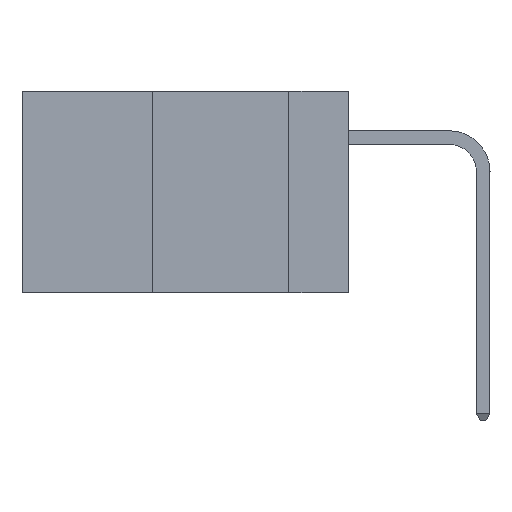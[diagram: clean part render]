
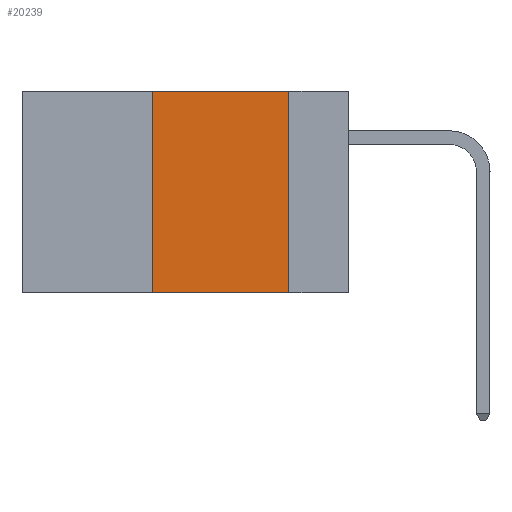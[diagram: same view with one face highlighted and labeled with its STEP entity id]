
A CAD part, left-side view. The second image highlights one B-rep face of the part: STEP entity #20239.
In plain terms, the highlighted planar face has unit normal (-1, 0, 0).
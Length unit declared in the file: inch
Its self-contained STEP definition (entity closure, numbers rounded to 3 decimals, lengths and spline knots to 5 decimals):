
#16 = CARTESIAN_POINT ( 'NONE',  ( 0., 0.11, 0. ) ) ;
#1268 = ORIENTED_EDGE ( 'NONE', *, *, #2205, .T. ) ;
#1293 = CARTESIAN_POINT ( 'NONE',  ( 0., 0.6, 0. ) ) ;
#1580 = EDGE_CURVE ( 'NONE', #20845, #8998, #15864, .T. ) ;
#2205 = EDGE_CURVE ( 'NONE', #19623, #19087, #8389, .T. ) ;
#2544 = EDGE_LOOP ( 'NONE', ( #24958, #12307, #13071, #1268 ) ) ;
#2777 = VECTOR ( 'NONE', #11764, 39.37008 ) ;
#3523 = DIRECTION ( 'NONE',  ( 0., 0., -1. ) ) ;
#3656 = PLANE ( 'NONE',  #23355 ) ;
#4199 = VECTOR ( 'NONE', #5696, 39.37008 ) ;
#5696 = DIRECTION ( 'NONE',  ( 0., -1., 0. ) ) ;
#7130 = EDGE_CURVE ( 'NONE', #8998, #19087, #12029, .T. ) ;
#8389 = LINE ( 'NONE', #16970, #13933 ) ;
#8667 = CARTESIAN_POINT ( 'NONE',  ( 0., 0.11, -0.37 ) ) ;
#8998 = VERTEX_POINT ( 'NONE', #13156 ) ;
#10999 = CARTESIAN_POINT ( 'NONE',  ( 0., 0.36, 0. ) ) ;
#11764 = DIRECTION ( 'NONE',  ( 0., 0., -1. ) ) ;
#12029 = LINE ( 'NONE', #16, #2777 ) ;
#12307 = ORIENTED_EDGE ( 'NONE', *, *, #1580, .F. ) ;
#13071 = ORIENTED_EDGE ( 'NONE', *, *, #18380, .F. ) ;
#13110 = DIRECTION ( 'NONE',  ( 0., 0., 1. ) ) ;
#13156 = CARTESIAN_POINT ( 'NONE',  ( 0., 0.11, 0. ) ) ;
#13695 = FACE_OUTER_BOUND ( 'NONE', #2544, .T. ) ;
#13933 = VECTOR ( 'NONE', #20390, 39.37008 ) ;
#14174 = CARTESIAN_POINT ( 'NONE',  ( 0., 0.36, -0.37 ) ) ;
#15101 = CARTESIAN_POINT ( 'NONE',  ( 0., 0.36, 0. ) ) ;
#15864 = LINE ( 'NONE', #25750, #4199 ) ;
#16970 = CARTESIAN_POINT ( 'NONE',  ( 0., 0.6, -0.37 ) ) ;
#18380 = EDGE_CURVE ( 'NONE', #19623, #20845, #18792, .T. ) ;
#18792 = LINE ( 'NONE', #15101, #25883 ) ;
#19087 = VERTEX_POINT ( 'NONE', #8667 ) ;
#19623 = VERTEX_POINT ( 'NONE', #14174 ) ;
#20239 = ADVANCED_FACE ( 'NONE', ( #13695 ), #3656, .F. ) ;
#20390 = DIRECTION ( 'NONE',  ( 0., -1., 0. ) ) ;
#20845 = VERTEX_POINT ( 'NONE', #10999 ) ;
#23355 = AXIS2_PLACEMENT_3D ( 'NONE', #1293, #23844, #3523 ) ;
#23844 = DIRECTION ( 'NONE',  ( 1., 0., 0. ) ) ;
#24958 = ORIENTED_EDGE ( 'NONE', *, *, #7130, .F. ) ;
#25750 = CARTESIAN_POINT ( 'NONE',  ( 0., 0.6, 0. ) ) ;
#25883 = VECTOR ( 'NONE', #13110, 39.37008 ) ;
